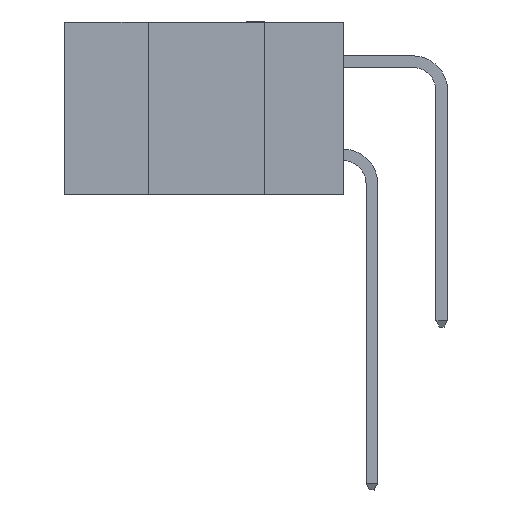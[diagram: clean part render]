
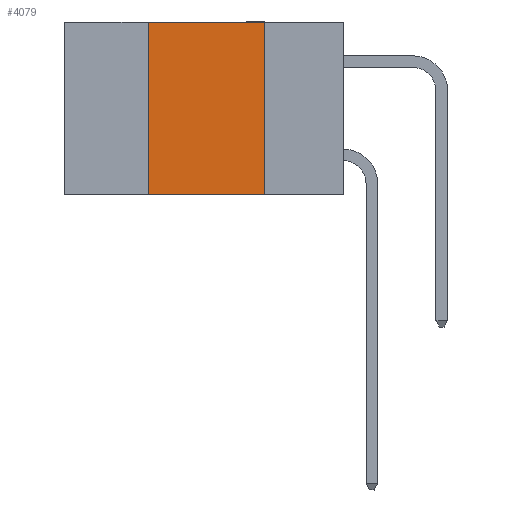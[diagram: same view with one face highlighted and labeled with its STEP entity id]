
A CAD part, left-side view. The second image highlights one B-rep face of the part: STEP entity #4079.
In plain terms, the highlighted planar face has unit normal (-1, 0, 0).
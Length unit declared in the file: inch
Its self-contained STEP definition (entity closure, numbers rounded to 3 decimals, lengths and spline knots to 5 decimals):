
#112 = CARTESIAN_POINT ( 'NONE',  ( 0., 0.6, 0. ) ) ;
#1298 = PLANE ( 'NONE',  #7159 ) ;
#1340 = CARTESIAN_POINT ( 'NONE',  ( 0., 0.42, -0.37 ) ) ;
#1675 = VECTOR ( 'NONE', #15938, 39.37008 ) ;
#3034 = VECTOR ( 'NONE', #6796, 39.37008 ) ;
#3623 = CARTESIAN_POINT ( 'NONE',  ( 0., 0.42, 0. ) ) ;
#3884 = LINE ( 'NONE', #3623, #10280 ) ;
#4079 = ADVANCED_FACE ( 'NONE', ( #13597 ), #1298, .F. ) ;
#4651 = CARTESIAN_POINT ( 'NONE',  ( 0., 0.17, 0. ) ) ;
#4745 = DIRECTION ( 'NONE',  ( 0., -1., 0. ) ) ;
#4790 = ORIENTED_EDGE ( 'NONE', *, *, #13661, .F. ) ;
#4945 = DIRECTION ( 'NONE',  ( 0., 0., 1. ) ) ;
#4996 = ORIENTED_EDGE ( 'NONE', *, *, #13873, .F. ) ;
#5020 = ORIENTED_EDGE ( 'NONE', *, *, #12830, .F. ) ;
#5124 = ORIENTED_EDGE ( 'NONE', *, *, #12013, .T. ) ;
#5534 = CARTESIAN_POINT ( 'NONE',  ( 0., 0.17, 0. ) ) ;
#5545 = VERTEX_POINT ( 'NONE', #1340 ) ;
#5885 = VECTOR ( 'NONE', #4745, 39.37008 ) ;
#6628 = CARTESIAN_POINT ( 'NONE',  ( 0., 0.17, -0.37 ) ) ;
#6796 = DIRECTION ( 'NONE',  ( 0., 0., -1. ) ) ;
#7045 = CARTESIAN_POINT ( 'NONE',  ( 0., 0.42, 0. ) ) ;
#7159 = AXIS2_PLACEMENT_3D ( 'NONE', #112, #14777, #8181 ) ;
#7219 = CARTESIAN_POINT ( 'NONE',  ( 0., 0.6, 0. ) ) ;
#8181 = DIRECTION ( 'NONE',  ( 0., 0., -1. ) ) ;
#9927 = VERTEX_POINT ( 'NONE', #4651 ) ;
#10280 = VECTOR ( 'NONE', #4945, 39.37008 ) ;
#10327 = VERTEX_POINT ( 'NONE', #6628 ) ;
#11224 = VERTEX_POINT ( 'NONE', #7045 ) ;
#11825 = LINE ( 'NONE', #14670, #1675 ) ;
#12013 = EDGE_CURVE ( 'NONE', #5545, #10327, #11825, .T. ) ;
#12830 = EDGE_CURVE ( 'NONE', #5545, #11224, #3884, .T. ) ;
#13091 = LINE ( 'NONE', #5534, #3034 ) ;
#13274 = LINE ( 'NONE', #7219, #5885 ) ;
#13597 = FACE_OUTER_BOUND ( 'NONE', #13671, .T. ) ;
#13661 = EDGE_CURVE ( 'NONE', #9927, #10327, #13091, .T. ) ;
#13671 = EDGE_LOOP ( 'NONE', ( #4790, #4996, #5020, #5124 ) ) ;
#13873 = EDGE_CURVE ( 'NONE', #11224, #9927, #13274, .T. ) ;
#14670 = CARTESIAN_POINT ( 'NONE',  ( 0., 0.6, -0.37 ) ) ;
#14777 = DIRECTION ( 'NONE',  ( 1., 0., 0. ) ) ;
#15938 = DIRECTION ( 'NONE',  ( 0., -1., 0. ) ) ;
